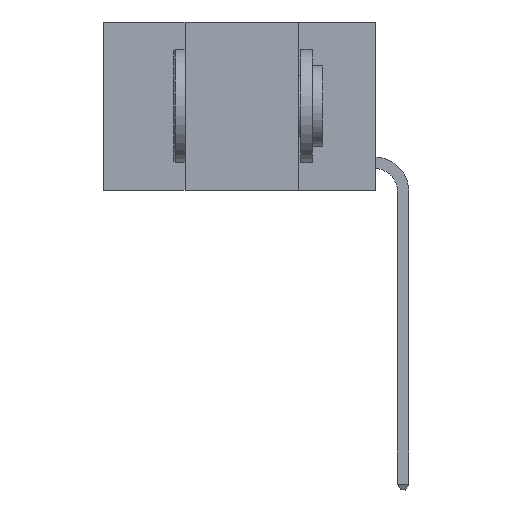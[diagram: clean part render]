
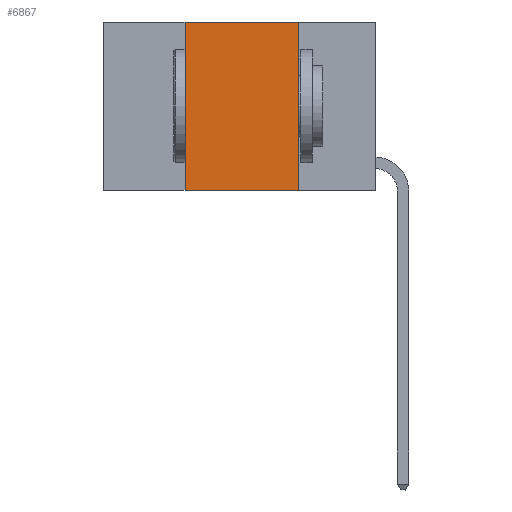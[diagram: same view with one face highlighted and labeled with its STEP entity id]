
A CAD part, left-side view. The second image highlights one B-rep face of the part: STEP entity #6867.
In plain terms, the highlighted planar face has unit normal (-1, 0, 0).
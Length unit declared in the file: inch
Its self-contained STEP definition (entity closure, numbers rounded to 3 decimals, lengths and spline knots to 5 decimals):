
#573 = AXIS2_PLACEMENT_3D ( 'NONE', #8734, #6822, #21261 ) ;
#1689 = VECTOR ( 'NONE', #22941, 39.37008 ) ;
#2099 = CARTESIAN_POINT ( 'NONE',  ( 0., 0.17, 0. ) ) ;
#2908 = EDGE_CURVE ( 'NONE', #10023, #9926, #22097, .T. ) ;
#3828 = CARTESIAN_POINT ( 'NONE',  ( 0., 0.17, 0. ) ) ;
#4810 = EDGE_CURVE ( 'NONE', #23082, #16319, #26367, .T. ) ;
#5796 = ORIENTED_EDGE ( 'NONE', *, *, #21373, .F. ) ;
#6822 = DIRECTION ( 'NONE',  ( 1., 0., 0. ) ) ;
#6867 = ADVANCED_FACE ( 'NONE', ( #21526 ), #12825, .F. ) ;
#7921 = ORIENTED_EDGE ( 'NONE', *, *, #8542, .F. ) ;
#8494 = LINE ( 'NONE', #2099, #1689 ) ;
#8542 = EDGE_CURVE ( 'NONE', #16319, #9926, #8494, .T. ) ;
#8734 = CARTESIAN_POINT ( 'NONE',  ( 0., 0.6, 0. ) ) ;
#9066 = CARTESIAN_POINT ( 'NONE',  ( 0., 0.42, 0. ) ) ;
#9446 = LINE ( 'NONE', #19041, #15428 ) ;
#9926 = VERTEX_POINT ( 'NONE', #11044 ) ;
#10023 = VERTEX_POINT ( 'NONE', #19733 ) ;
#10053 = DIRECTION ( 'NONE',  ( 0., -1., 0. ) ) ;
#10126 = DIRECTION ( 'NONE',  ( 0., -1., 0. ) ) ;
#11044 = CARTESIAN_POINT ( 'NONE',  ( 0., 0.17, -0.37 ) ) ;
#11379 = DIRECTION ( 'NONE',  ( 0., 0., 1. ) ) ;
#12825 = PLANE ( 'NONE',  #573 ) ;
#15428 = VECTOR ( 'NONE', #11379, 39.37008 ) ;
#16319 = VERTEX_POINT ( 'NONE', #3828 ) ;
#17304 = ORIENTED_EDGE ( 'NONE', *, *, #2908, .T. ) ;
#19041 = CARTESIAN_POINT ( 'NONE',  ( 0., 0.42, 0. ) ) ;
#19143 = EDGE_LOOP ( 'NONE', ( #7921, #26438, #5796, #17304 ) ) ;
#19733 = CARTESIAN_POINT ( 'NONE',  ( 0., 0.42, -0.37 ) ) ;
#21198 = VECTOR ( 'NONE', #10126, 39.37008 ) ;
#21219 = VECTOR ( 'NONE', #10053, 39.37008 ) ;
#21261 = DIRECTION ( 'NONE',  ( 0., 0., -1. ) ) ;
#21373 = EDGE_CURVE ( 'NONE', #10023, #23082, #9446, .T. ) ;
#21526 = FACE_OUTER_BOUND ( 'NONE', #19143, .T. ) ;
#22097 = LINE ( 'NONE', #24269, #21198 ) ;
#22167 = CARTESIAN_POINT ( 'NONE',  ( 0., 0.6, 0. ) ) ;
#22941 = DIRECTION ( 'NONE',  ( 0., 0., -1. ) ) ;
#23082 = VERTEX_POINT ( 'NONE', #9066 ) ;
#24269 = CARTESIAN_POINT ( 'NONE',  ( 0., 0.6, -0.37 ) ) ;
#26367 = LINE ( 'NONE', #22167, #21219 ) ;
#26438 = ORIENTED_EDGE ( 'NONE', *, *, #4810, .F. ) ;
